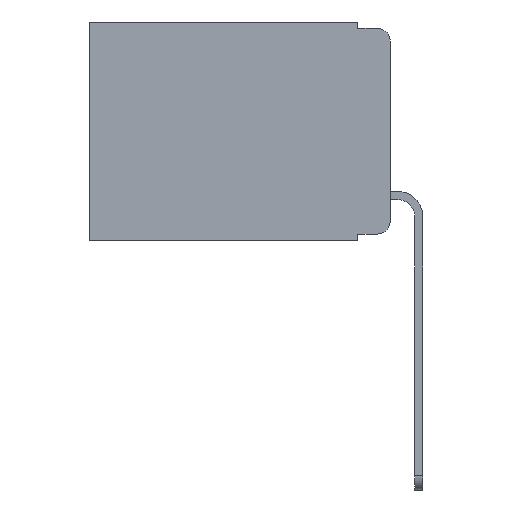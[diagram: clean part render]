
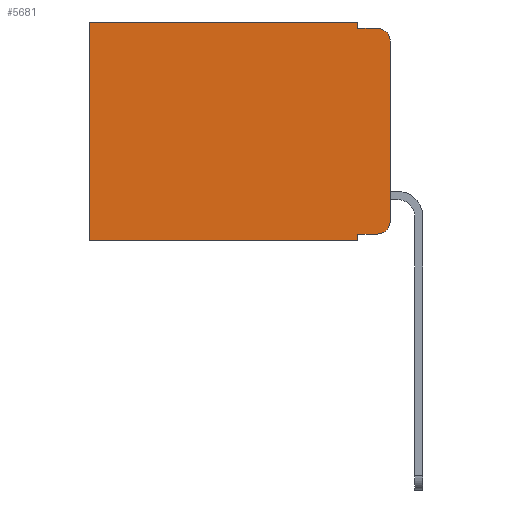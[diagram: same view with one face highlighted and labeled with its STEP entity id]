
A CAD part, left-side view. The second image highlights one B-rep face of the part: STEP entity #5681.
In plain terms, the highlighted planar face has unit normal (-1, 0, 0).
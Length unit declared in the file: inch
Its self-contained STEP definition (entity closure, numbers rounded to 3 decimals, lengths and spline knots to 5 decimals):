
#195 = DIRECTION ( 'NONE',  ( -1., 0., 0. ) ) ;
#382 = VERTEX_POINT ( 'NONE', #13949 ) ;
#685 = CARTESIAN_POINT ( 'NONE',  ( 0.298, 0.051, -0.343 ) ) ;
#777 = ORIENTED_EDGE ( 'NONE', *, *, #14257, .F. ) ;
#1352 = VECTOR ( 'NONE', #13966, 39.37008 ) ;
#1415 = CIRCLE ( 'NONE', #13680, 0.02 ) ;
#1483 = CARTESIAN_POINT ( 'NONE',  ( 0.298, 0., 0. ) ) ;
#1672 = CARTESIAN_POINT ( 'NONE',  ( 0.298, 0.473, 0. ) ) ;
#1778 = VECTOR ( 'NONE', #11496, 39.37008 ) ;
#2057 = VERTEX_POINT ( 'NONE', #685 ) ;
#2223 = LINE ( 'NONE', #9697, #12758 ) ;
#2556 = VECTOR ( 'NONE', #8676, 39.37008 ) ;
#3053 = ORIENTED_EDGE ( 'NONE', *, *, #7365, .T. ) ;
#3258 = CARTESIAN_POINT ( 'NONE',  ( 0.298, 0.051, -0.01 ) ) ;
#3721 = ORIENTED_EDGE ( 'NONE', *, *, #10924, .F. ) ;
#4388 = CARTESIAN_POINT ( 'NONE',  ( 0.298, 0.051, 0. ) ) ;
#4651 = CARTESIAN_POINT ( 'NONE',  ( 0.298, 0.02, -0.333 ) ) ;
#4780 = CARTESIAN_POINT ( 'NONE',  ( 0.298, 0.051, -0.333 ) ) ;
#4970 = ORIENTED_EDGE ( 'NONE', *, *, #11803, .F. ) ;
#5039 = LINE ( 'NONE', #17132, #11767 ) ;
#5681 = ADVANCED_FACE ( 'NONE', ( #7893 ), #7538, .F. ) ;
#5731 = VERTEX_POINT ( 'NONE', #3258 ) ;
#6299 = CARTESIAN_POINT ( 'NONE',  ( 0.298, 0.051, -0.333 ) ) ;
#6354 = CARTESIAN_POINT ( 'NONE',  ( 0.298, 0.473, 0. ) ) ;
#6474 = CARTESIAN_POINT ( 'NONE',  ( 0.298, 0.051, 0. ) ) ;
#6744 = LINE ( 'NONE', #1672, #1778 ) ;
#6746 = CARTESIAN_POINT ( 'NONE',  ( 0.298, 0.02, -0.313 ) ) ;
#6992 = VERTEX_POINT ( 'NONE', #14259 ) ;
#7200 = ORIENTED_EDGE ( 'NONE', *, *, #8381, .T. ) ;
#7365 = EDGE_CURVE ( 'NONE', #10182, #12573, #11542, .T. ) ;
#7467 = EDGE_CURVE ( 'NONE', #12188, #17126, #13113, .T. ) ;
#7538 = PLANE ( 'NONE',  #15933 ) ;
#7844 = AXIS2_PLACEMENT_3D ( 'NONE', #6746, #15583, #8140 ) ;
#7893 = FACE_OUTER_BOUND ( 'NONE', #12381, .T. ) ;
#8140 = DIRECTION ( 'NONE',  ( 0., 0., -1. ) ) ;
#8381 = EDGE_CURVE ( 'NONE', #12496, #12188, #15335, .T. ) ;
#8453 = DIRECTION ( 'NONE',  ( 0., -1., 0. ) ) ;
#8495 = DIRECTION ( 'NONE',  ( 0., 1., 0. ) ) ;
#8676 = DIRECTION ( 'NONE',  ( 0., 0., -1. ) ) ;
#8804 = LINE ( 'NONE', #13516, #15017 ) ;
#9125 = CARTESIAN_POINT ( 'NONE',  ( 0.298, 0.02, -0.03 ) ) ;
#9231 = CARTESIAN_POINT ( 'NONE',  ( 0.298, 0., 0. ) ) ;
#9252 = EDGE_CURVE ( 'NONE', #12496, #2057, #16958, .T. ) ;
#9697 = CARTESIAN_POINT ( 'NONE',  ( 0.298, 0.051, 0. ) ) ;
#10051 = EDGE_CURVE ( 'NONE', #12573, #382, #6744, .T. ) ;
#10123 = DIRECTION ( 'NONE',  ( 0., 0., -1. ) ) ;
#10182 = VERTEX_POINT ( 'NONE', #6474 ) ;
#10389 = DIRECTION ( 'NONE',  ( 0., 0., -1. ) ) ;
#10924 = EDGE_CURVE ( 'NONE', #10182, #5731, #2223, .T. ) ;
#10983 = DIRECTION ( 'NONE',  ( 0., 0., -1. ) ) ;
#11496 = DIRECTION ( 'NONE',  ( 0., 0., -1. ) ) ;
#11527 = VECTOR ( 'NONE', #8495, 39.37008 ) ;
#11542 = LINE ( 'NONE', #9231, #14438 ) ;
#11767 = VECTOR ( 'NONE', #17182, 39.37008 ) ;
#11803 = EDGE_CURVE ( 'NONE', #5731, #6992, #8804, .T. ) ;
#12188 = VERTEX_POINT ( 'NONE', #4651 ) ;
#12354 = VERTEX_POINT ( 'NONE', #13814 ) ;
#12381 = EDGE_LOOP ( 'NONE', ( #777, #13200, #4970, #3721, #3053, #14091, #15638, #14715, #7200, #15931 ) ) ;
#12496 = VERTEX_POINT ( 'NONE', #6299 ) ;
#12573 = VERTEX_POINT ( 'NONE', #6354 ) ;
#12601 = EDGE_CURVE ( 'NONE', #12354, #6992, #1415, .T. ) ;
#12758 = VECTOR ( 'NONE', #10983, 39.37008 ) ;
#13113 = CIRCLE ( 'NONE', #7844, 0.02 ) ;
#13200 = ORIENTED_EDGE ( 'NONE', *, *, #12601, .T. ) ;
#13516 = CARTESIAN_POINT ( 'NONE',  ( 0.298, 0.051, -0.01 ) ) ;
#13680 = AXIS2_PLACEMENT_3D ( 'NONE', #9125, #195, #10389 ) ;
#13814 = CARTESIAN_POINT ( 'NONE',  ( 0.298, 0., -0.03 ) ) ;
#13843 = DIRECTION ( 'NONE',  ( 1., 0., 0. ) ) ;
#13949 = CARTESIAN_POINT ( 'NONE',  ( 0.298, 0.473, -0.343 ) ) ;
#13966 = DIRECTION ( 'NONE',  ( 0., -1., 0. ) ) ;
#14091 = ORIENTED_EDGE ( 'NONE', *, *, #10051, .T. ) ;
#14257 = EDGE_CURVE ( 'NONE', #12354, #17126, #5039, .T. ) ;
#14259 = CARTESIAN_POINT ( 'NONE',  ( 0.298, 0.02, -0.01 ) ) ;
#14438 = VECTOR ( 'NONE', #15429, 39.37008 ) ;
#14715 = ORIENTED_EDGE ( 'NONE', *, *, #9252, .F. ) ;
#14787 = LINE ( 'NONE', #15906, #11527 ) ;
#15017 = VECTOR ( 'NONE', #8453, 39.37008 ) ;
#15335 = LINE ( 'NONE', #4780, #1352 ) ;
#15429 = DIRECTION ( 'NONE',  ( 0., 1., 0. ) ) ;
#15550 = EDGE_CURVE ( 'NONE', #2057, #382, #14787, .T. ) ;
#15583 = DIRECTION ( 'NONE',  ( -1., 0., 0. ) ) ;
#15638 = ORIENTED_EDGE ( 'NONE', *, *, #15550, .F. ) ;
#15906 = CARTESIAN_POINT ( 'NONE',  ( 0.298, 0., -0.343 ) ) ;
#15931 = ORIENTED_EDGE ( 'NONE', *, *, #7467, .T. ) ;
#15933 = AXIS2_PLACEMENT_3D ( 'NONE', #1483, #13843, #10123 ) ;
#16958 = LINE ( 'NONE', #4388, #2556 ) ;
#17126 = VERTEX_POINT ( 'NONE', #17480 ) ;
#17132 = CARTESIAN_POINT ( 'NONE',  ( 0.298, 0., 0. ) ) ;
#17182 = DIRECTION ( 'NONE',  ( 0., 0., -1. ) ) ;
#17480 = CARTESIAN_POINT ( 'NONE',  ( 0.298, 0., -0.313 ) ) ;
